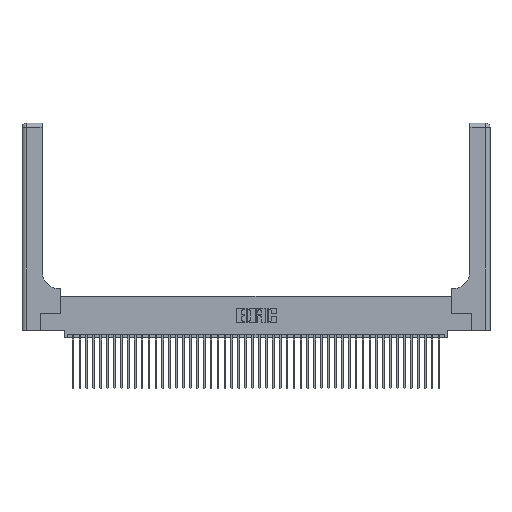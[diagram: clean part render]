
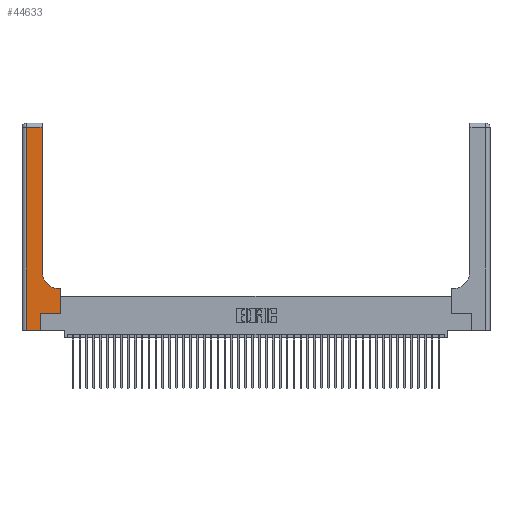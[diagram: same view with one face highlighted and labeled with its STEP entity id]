
A CAD part, top view. The second image highlights one B-rep face of the part: STEP entity #44633.
In plain terms, the highlighted planar face has unit normal (0, 0, 1).
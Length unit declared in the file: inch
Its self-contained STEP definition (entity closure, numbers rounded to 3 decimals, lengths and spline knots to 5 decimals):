
#701 = VECTOR ( 'NONE', #17371, 39.37008 ) ;
#816 = DIRECTION ( 'NONE',  ( 0., 1., 0. ) ) ;
#892 = VERTEX_POINT ( 'NONE', #20092 ) ;
#2911 = CARTESIAN_POINT ( 'NONE',  ( 0.269, 0., 0.37 ) ) ;
#2919 = CIRCLE ( 'NONE', #28415, 0.25 ) ;
#3093 = PLANE ( 'NONE',  #23625 ) ;
#3590 = EDGE_CURVE ( 'NONE', #5638, #17733, #19886, .T. ) ;
#3632 = EDGE_CURVE ( 'NONE', #33623, #5352, #45832, .T. ) ;
#3692 = CARTESIAN_POINT ( 'NONE',  ( 0.06, 0., 0.37 ) ) ;
#4501 = CARTESIAN_POINT ( 'NONE',  ( 0.2915, 3., 0.37 ) ) ;
#5352 = VERTEX_POINT ( 'NONE', #35099 ) ;
#5483 = DIRECTION ( 'NONE',  ( -1., 0., 0. ) ) ;
#5638 = VERTEX_POINT ( 'NONE', #33034 ) ;
#6641 = ORIENTED_EDGE ( 'NONE', *, *, #10812, .T. ) ;
#7163 = CARTESIAN_POINT ( 'NONE',  ( 0., 0., 0.37 ) ) ;
#7476 = ORIENTED_EDGE ( 'NONE', *, *, #3632, .T. ) ;
#8016 = VECTOR ( 'NONE', #14982, 39.37008 ) ;
#9166 = LINE ( 'NONE', #39744, #8016 ) ;
#9636 = EDGE_CURVE ( 'NONE', #31661, #42723, #40300, .T. ) ;
#9947 = EDGE_CURVE ( 'NONE', #25119, #33623, #9166, .T. ) ;
#10317 = EDGE_CURVE ( 'NONE', #5352, #31428, #2919, .T. ) ;
#10351 = DIRECTION ( 'NONE',  ( -1., 0., 0. ) ) ;
#10812 = EDGE_CURVE ( 'NONE', #31428, #892, #30255, .T. ) ;
#11328 = VECTOR ( 'NONE', #816, 39.37008 ) ;
#11860 = VECTOR ( 'NONE', #32074, 39.37008 ) ;
#12009 = VECTOR ( 'NONE', #15316, 39.37008 ) ;
#12214 = CARTESIAN_POINT ( 'NONE',  ( 0.2915, 0.85, 0.37 ) ) ;
#13221 = DIRECTION ( 'NONE',  ( 0., 0., -1. ) ) ;
#13603 = DIRECTION ( 'NONE',  ( 0., -1., 0. ) ) ;
#13959 = DIRECTION ( 'NONE',  ( -1., 0., 0. ) ) ;
#14982 = DIRECTION ( 'NONE',  ( 0., 1., 0. ) ) ;
#15316 = DIRECTION ( 'NONE',  ( 1., 0., 0. ) ) ;
#15907 = FACE_OUTER_BOUND ( 'NONE', #26422, .T. ) ;
#17371 = DIRECTION ( 'NONE',  ( 0., 1., 0. ) ) ;
#17609 = EDGE_CURVE ( 'NONE', #17733, #25119, #32030, .T. ) ;
#17733 = VERTEX_POINT ( 'NONE', #37297 ) ;
#18097 = ORIENTED_EDGE ( 'NONE', *, *, #10317, .T. ) ;
#19277 = VECTOR ( 'NONE', #13603, 39.37008 ) ;
#19886 = LINE ( 'NONE', #2911, #701 ) ;
#20092 = CARTESIAN_POINT ( 'NONE',  ( 0.2915, 2.94, 0.37 ) ) ;
#20734 = EDGE_CURVE ( 'NONE', #892, #31661, #34806, .T. ) ;
#22054 = ORIENTED_EDGE ( 'NONE', *, *, #3590, .T. ) ;
#23625 = AXIS2_PLACEMENT_3D ( 'NONE', #28107, #31642, #10351 ) ;
#24076 = CARTESIAN_POINT ( 'NONE',  ( 0.06, 2.94, 0.37 ) ) ;
#25119 = VERTEX_POINT ( 'NONE', #34934 ) ;
#25426 = VECTOR ( 'NONE', #5483, 39.37008 ) ;
#26422 = EDGE_LOOP ( 'NONE', ( #6641, #33234, #34390, #29317, #22054, #40261, #36357, #7476, #18097 ) ) ;
#28107 = CARTESIAN_POINT ( 'NONE',  ( 0., 3., 0.37 ) ) ;
#28415 = AXIS2_PLACEMENT_3D ( 'NONE', #34464, #13221, #38009 ) ;
#29317 = ORIENTED_EDGE ( 'NONE', *, *, #33654, .T. ) ;
#30255 = LINE ( 'NONE', #4501, #11328 ) ;
#31428 = VERTEX_POINT ( 'NONE', #12214 ) ;
#31621 = CARTESIAN_POINT ( 'NONE',  ( 0.2915, 0.6, 0.37 ) ) ;
#31642 = DIRECTION ( 'NONE',  ( 0., 0., -1. ) ) ;
#31661 = VERTEX_POINT ( 'NONE', #24076 ) ;
#32030 = LINE ( 'NONE', #33115, #12009 ) ;
#32074 = DIRECTION ( 'NONE',  ( 1., 0., 0. ) ) ;
#33034 = CARTESIAN_POINT ( 'NONE',  ( 0.269, 0., 0.37 ) ) ;
#33115 = CARTESIAN_POINT ( 'NONE',  ( 0.269, 0.25, 0.37 ) ) ;
#33234 = ORIENTED_EDGE ( 'NONE', *, *, #20734, .T. ) ;
#33623 = VERTEX_POINT ( 'NONE', #45941 ) ;
#33654 = EDGE_CURVE ( 'NONE', #42723, #5638, #39057, .T. ) ;
#33813 = CARTESIAN_POINT ( 'NONE',  ( 0., 2.94, 0.37 ) ) ;
#34390 = ORIENTED_EDGE ( 'NONE', *, *, #9636, .T. ) ;
#34464 = CARTESIAN_POINT ( 'NONE',  ( 0.5415, 0.85, 0.37 ) ) ;
#34806 = LINE ( 'NONE', #33813, #25426 ) ;
#34934 = CARTESIAN_POINT ( 'NONE',  ( 0.5585, 0.25, 0.37 ) ) ;
#35099 = CARTESIAN_POINT ( 'NONE',  ( 0.5415, 0.6, 0.37 ) ) ;
#36357 = ORIENTED_EDGE ( 'NONE', *, *, #9947, .T. ) ;
#36450 = VECTOR ( 'NONE', #13959, 39.37008 ) ;
#37297 = CARTESIAN_POINT ( 'NONE',  ( 0.269, 0.25, 0.37 ) ) ;
#38009 = DIRECTION ( 'NONE',  ( 1., 0., 0. ) ) ;
#38375 = CARTESIAN_POINT ( 'NONE',  ( 0.06, 3., 0.37 ) ) ;
#39057 = LINE ( 'NONE', #7163, #11860 ) ;
#39744 = CARTESIAN_POINT ( 'NONE',  ( 0.5585, 0.25, 0.37 ) ) ;
#40261 = ORIENTED_EDGE ( 'NONE', *, *, #17609, .T. ) ;
#40300 = LINE ( 'NONE', #38375, #19277 ) ;
#42723 = VERTEX_POINT ( 'NONE', #3692 ) ;
#44633 = ADVANCED_FACE ( 'NONE', ( #15907 ), #3093, .F. ) ;
#45832 = LINE ( 'NONE', #31621, #36450 ) ;
#45941 = CARTESIAN_POINT ( 'NONE',  ( 0.5585, 0.6, 0.37 ) ) ;
